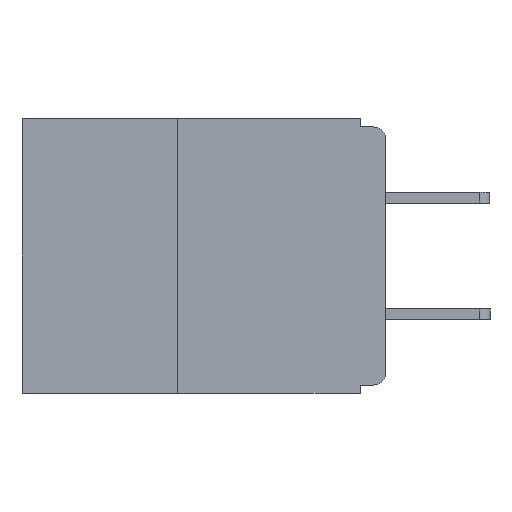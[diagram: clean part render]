
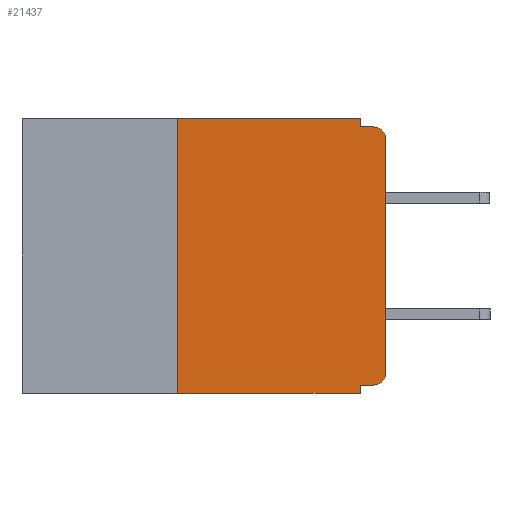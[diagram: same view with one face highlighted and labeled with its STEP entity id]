
A CAD part, left-side view. The second image highlights one B-rep face of the part: STEP entity #21437.
In plain terms, the highlighted planar face has unit normal (-1, 0, 0).
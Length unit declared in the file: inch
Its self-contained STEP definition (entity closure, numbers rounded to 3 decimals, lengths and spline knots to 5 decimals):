
#25 = CARTESIAN_POINT ( 'NONE',  ( 0., 0.031, -0.01 ) ) ;
#578 = ORIENTED_EDGE ( 'NONE', *, *, #12519, .T. ) ;
#802 = DIRECTION ( 'NONE',  ( 0., 0., -1. ) ) ;
#1099 = ORIENTED_EDGE ( 'NONE', *, *, #10843, .F. ) ;
#1336 = CARTESIAN_POINT ( 'NONE',  ( 0., 0.25, 0. ) ) ;
#1563 = ORIENTED_EDGE ( 'NONE', *, *, #5176, .F. ) ;
#1580 = VERTEX_POINT ( 'NONE', #30234 ) ;
#1688 = ORIENTED_EDGE ( 'NONE', *, *, #23871, .T. ) ;
#1851 = VECTOR ( 'NONE', #8919, 39.37008 ) ;
#2540 = LINE ( 'NONE', #3185, #27783 ) ;
#3185 = CARTESIAN_POINT ( 'NONE',  ( 0., 0.437, 0. ) ) ;
#3554 = LINE ( 'NONE', #14944, #28775 ) ;
#3752 = CARTESIAN_POINT ( 'NONE',  ( 0., 0.25, -0.33 ) ) ;
#5081 = DIRECTION ( 'NONE',  ( 0., 0., 1. ) ) ;
#5176 = EDGE_CURVE ( 'NONE', #16055, #28911, #20810, .T. ) ;
#5185 = DIRECTION ( 'NONE',  ( 0., -1., 0. ) ) ;
#5281 = CARTESIAN_POINT ( 'NONE',  ( 0., 0.437, 0. ) ) ;
#5932 = LINE ( 'NONE', #25510, #18222 ) ;
#6699 = LINE ( 'NONE', #10683, #26299 ) ;
#6755 = EDGE_LOOP ( 'NONE', ( #29589, #18439, #25292, #26852, #27425, #28475, #578, #1099, #1563, #1688 ) ) ;
#6897 = CARTESIAN_POINT ( 'NONE',  ( 0., 0., -0.32 ) ) ;
#7164 = VERTEX_POINT ( 'NONE', #25 ) ;
#7717 = DIRECTION ( 'NONE',  ( 0., 0., -1. ) ) ;
#7792 = VERTEX_POINT ( 'NONE', #1336 ) ;
#8460 = CARTESIAN_POINT ( 'NONE',  ( 0., 0.015, -0.32 ) ) ;
#8472 = CARTESIAN_POINT ( 'NONE',  ( 0., 0., -0.305 ) ) ;
#8919 = DIRECTION ( 'NONE',  ( 0., -1., 0. ) ) ;
#9825 = CARTESIAN_POINT ( 'NONE',  ( 0., 0.015, -0.025 ) ) ;
#10209 = CIRCLE ( 'NONE', #28735, 0.015 ) ;
#10683 = CARTESIAN_POINT ( 'NONE',  ( 0., 0.031, -0.33 ) ) ;
#10778 = EDGE_CURVE ( 'NONE', #7792, #15087, #2540, .T. ) ;
#10843 = EDGE_CURVE ( 'NONE', #28911, #15732, #6699, .T. ) ;
#11502 = CARTESIAN_POINT ( 'NONE',  ( 0., 0.031, 0. ) ) ;
#11624 = VERTEX_POINT ( 'NONE', #3752 ) ;
#11705 = DIRECTION ( 'NONE',  ( 0., 1., 0. ) ) ;
#12022 = VECTOR ( 'NONE', #21648, 39.37008 ) ;
#12313 = DIRECTION ( 'NONE',  ( 0., 0., -1. ) ) ;
#12519 = EDGE_CURVE ( 'NONE', #11624, #15732, #3554, .T. ) ;
#12956 = CARTESIAN_POINT ( 'NONE',  ( 0., 0.031, -0.32 ) ) ;
#13705 = VERTEX_POINT ( 'NONE', #8472 ) ;
#14119 = FACE_OUTER_BOUND ( 'NONE', #6755, .T. ) ;
#14862 = VERTEX_POINT ( 'NONE', #30085 ) ;
#14944 = CARTESIAN_POINT ( 'NONE',  ( 0., 0.437, -0.33 ) ) ;
#15043 = EDGE_CURVE ( 'NONE', #7164, #1580, #27163, .T. ) ;
#15052 = VECTOR ( 'NONE', #11705, 39.37008 ) ;
#15087 = VERTEX_POINT ( 'NONE', #11502 ) ;
#15360 = DIRECTION ( 'NONE',  ( 0., -1., 0. ) ) ;
#15491 = DIRECTION ( 'NONE',  ( -1., 0., 0. ) ) ;
#15567 = DIRECTION ( 'NONE',  ( 0., 0., -1. ) ) ;
#15732 = VERTEX_POINT ( 'NONE', #26637 ) ;
#15843 = EDGE_CURVE ( 'NONE', #11624, #7792, #17145, .T. ) ;
#16055 = VERTEX_POINT ( 'NONE', #8460 ) ;
#17145 = LINE ( 'NONE', #19776, #30067 ) ;
#17471 = EDGE_CURVE ( 'NONE', #15087, #7164, #18561, .T. ) ;
#17497 = PLANE ( 'NONE',  #21069 ) ;
#18222 = VECTOR ( 'NONE', #27919, 39.37008 ) ;
#18439 = ORIENTED_EDGE ( 'NONE', *, *, #28737, .T. ) ;
#18561 = LINE ( 'NONE', #31159, #12022 ) ;
#19776 = CARTESIAN_POINT ( 'NONE',  ( 0., 0.25, -0.33 ) ) ;
#20810 = LINE ( 'NONE', #6897, #15052 ) ;
#21069 = AXIS2_PLACEMENT_3D ( 'NONE', #5281, #22485, #7717 ) ;
#21437 = ADVANCED_FACE ( 'NONE', ( #14119 ), #17497, .F. ) ;
#21648 = DIRECTION ( 'NONE',  ( 0., 0., -1. ) ) ;
#22485 = DIRECTION ( 'NONE',  ( 1., 0., 0. ) ) ;
#23273 = EDGE_CURVE ( 'NONE', #13705, #14862, #5932, .T. ) ;
#23671 = CARTESIAN_POINT ( 'NONE',  ( 0., 0., -0.01 ) ) ;
#23871 = EDGE_CURVE ( 'NONE', #16055, #13705, #26625, .T. ) ;
#24395 = AXIS2_PLACEMENT_3D ( 'NONE', #30045, #15491, #802 ) ;
#25292 = ORIENTED_EDGE ( 'NONE', *, *, #15043, .F. ) ;
#25510 = CARTESIAN_POINT ( 'NONE',  ( 0., 0., 0. ) ) ;
#26299 = VECTOR ( 'NONE', #15567, 39.37008 ) ;
#26625 = CIRCLE ( 'NONE', #24395, 0.015 ) ;
#26637 = CARTESIAN_POINT ( 'NONE',  ( 0., 0.031, -0.33 ) ) ;
#26852 = ORIENTED_EDGE ( 'NONE', *, *, #17471, .F. ) ;
#27018 = DIRECTION ( 'NONE',  ( -1., 0., 0. ) ) ;
#27163 = LINE ( 'NONE', #23671, #1851 ) ;
#27425 = ORIENTED_EDGE ( 'NONE', *, *, #10778, .F. ) ;
#27783 = VECTOR ( 'NONE', #15360, 39.37008 ) ;
#27919 = DIRECTION ( 'NONE',  ( 0., 0., 1. ) ) ;
#28475 = ORIENTED_EDGE ( 'NONE', *, *, #15843, .F. ) ;
#28735 = AXIS2_PLACEMENT_3D ( 'NONE', #9825, #27018, #12313 ) ;
#28737 = EDGE_CURVE ( 'NONE', #14862, #1580, #10209, .T. ) ;
#28775 = VECTOR ( 'NONE', #5185, 39.37008 ) ;
#28911 = VERTEX_POINT ( 'NONE', #12956 ) ;
#29589 = ORIENTED_EDGE ( 'NONE', *, *, #23273, .T. ) ;
#30045 = CARTESIAN_POINT ( 'NONE',  ( 0., 0.015, -0.305 ) ) ;
#30067 = VECTOR ( 'NONE', #5081, 39.37008 ) ;
#30085 = CARTESIAN_POINT ( 'NONE',  ( 0., 0., -0.025 ) ) ;
#30234 = CARTESIAN_POINT ( 'NONE',  ( 0., 0.015, -0.01 ) ) ;
#31159 = CARTESIAN_POINT ( 'NONE',  ( 0., 0.031, 0. ) ) ;
